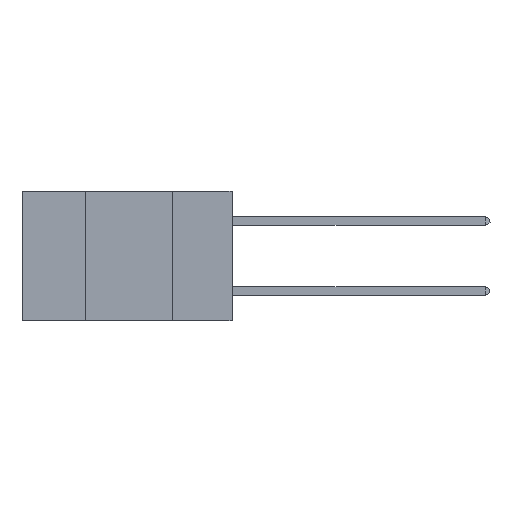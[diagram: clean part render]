
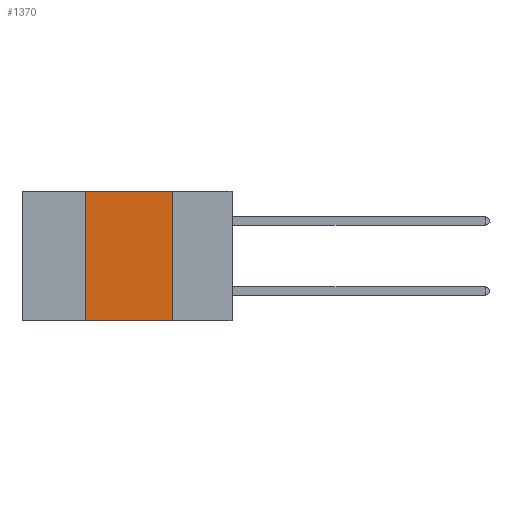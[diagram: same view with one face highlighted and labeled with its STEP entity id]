
A CAD part, left-side view. The second image highlights one B-rep face of the part: STEP entity #1370.
In plain terms, the highlighted planar face has unit normal (-1, 0, 0).
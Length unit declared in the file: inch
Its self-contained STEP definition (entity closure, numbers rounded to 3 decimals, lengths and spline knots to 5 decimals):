
#483 = VERTEX_POINT ( 'NONE', #16171 ) ;
#568 = DIRECTION ( 'NONE',  ( 0., 0., -1. ) ) ;
#612 = EDGE_CURVE ( 'NONE', #483, #12660, #13945, .T. ) ;
#1093 = DIRECTION ( 'NONE',  ( 0., 0., -1. ) ) ;
#1162 = CARTESIAN_POINT ( 'NONE',  ( 0., 0.42, -0.37 ) ) ;
#1370 = ADVANCED_FACE ( 'NONE', ( #13111 ), #17351, .F. ) ;
#1907 = CARTESIAN_POINT ( 'NONE',  ( 0., 0.17, 0. ) ) ;
#1974 = ORIENTED_EDGE ( 'NONE', *, *, #2181, .T. ) ;
#2181 = EDGE_CURVE ( 'NONE', #12053, #12660, #16110, .T. ) ;
#2616 = ORIENTED_EDGE ( 'NONE', *, *, #4568, .F. ) ;
#2659 = DIRECTION ( 'NONE',  ( 0., 0., 1. ) ) ;
#2780 = ORIENTED_EDGE ( 'NONE', *, *, #612, .F. ) ;
#4568 = EDGE_CURVE ( 'NONE', #10729, #483, #8533, .T. ) ;
#4944 = CARTESIAN_POINT ( 'NONE',  ( 0., 0.6, 0. ) ) ;
#5050 = VECTOR ( 'NONE', #9184, 39.37008 ) ;
#6425 = VECTOR ( 'NONE', #2659, 39.37008 ) ;
#6508 = LINE ( 'NONE', #16133, #6425 ) ;
#7755 = ORIENTED_EDGE ( 'NONE', *, *, #13650, .F. ) ;
#8027 = CARTESIAN_POINT ( 'NONE',  ( 0., 0.6, -0.37 ) ) ;
#8332 = CARTESIAN_POINT ( 'NONE',  ( 0., 0.17, -0.37 ) ) ;
#8533 = LINE ( 'NONE', #14098, #13944 ) ;
#9184 = DIRECTION ( 'NONE',  ( 0., -1., 0. ) ) ;
#10689 = EDGE_LOOP ( 'NONE', ( #2780, #2616, #7755, #1974 ) ) ;
#10729 = VERTEX_POINT ( 'NONE', #14636 ) ;
#12053 = VERTEX_POINT ( 'NONE', #1162 ) ;
#12393 = VECTOR ( 'NONE', #568, 39.37008 ) ;
#12660 = VERTEX_POINT ( 'NONE', #8332 ) ;
#12915 = DIRECTION ( 'NONE',  ( 0., -1., 0. ) ) ;
#13111 = FACE_OUTER_BOUND ( 'NONE', #10689, .T. ) ;
#13650 = EDGE_CURVE ( 'NONE', #12053, #10729, #6508, .T. ) ;
#13944 = VECTOR ( 'NONE', #12915, 39.37008 ) ;
#13945 = LINE ( 'NONE', #1907, #12393 ) ;
#14098 = CARTESIAN_POINT ( 'NONE',  ( 0., 0.6, 0. ) ) ;
#14636 = CARTESIAN_POINT ( 'NONE',  ( 0., 0.42, 0. ) ) ;
#15072 = AXIS2_PLACEMENT_3D ( 'NONE', #4944, #17438, #1093 ) ;
#16110 = LINE ( 'NONE', #8027, #5050 ) ;
#16133 = CARTESIAN_POINT ( 'NONE',  ( 0., 0.42, 0. ) ) ;
#16171 = CARTESIAN_POINT ( 'NONE',  ( 0., 0.17, 0. ) ) ;
#17351 = PLANE ( 'NONE',  #15072 ) ;
#17438 = DIRECTION ( 'NONE',  ( 1., 0., 0. ) ) ;
